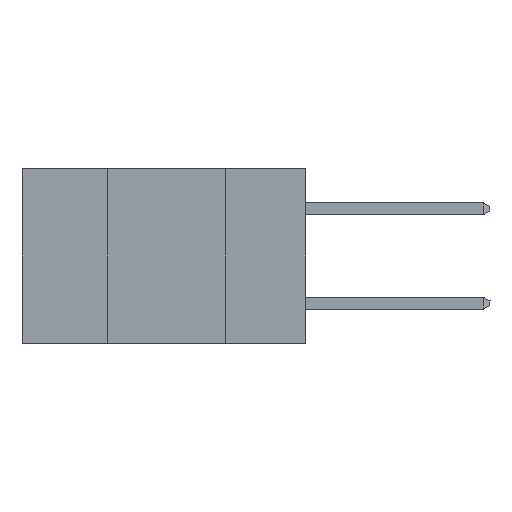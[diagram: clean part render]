
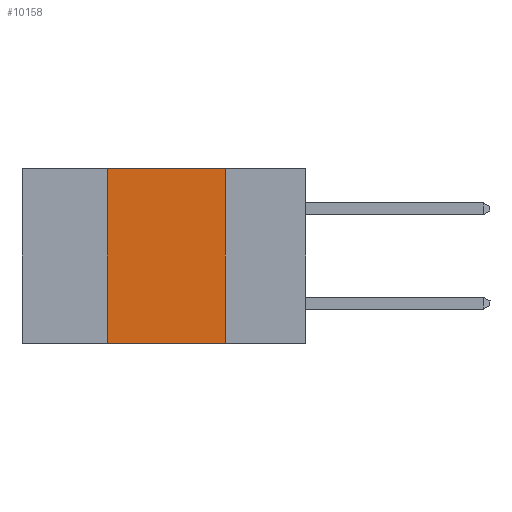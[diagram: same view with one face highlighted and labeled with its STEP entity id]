
A CAD part, left-side view. The second image highlights one B-rep face of the part: STEP entity #10158.
In plain terms, the highlighted planar face has unit normal (-1, 0, 0).
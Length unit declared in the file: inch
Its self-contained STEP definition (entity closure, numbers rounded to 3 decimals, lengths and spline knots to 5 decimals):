
#963 = DIRECTION ( 'NONE',  ( 0., 0., -1. ) ) ;
#1073 = VECTOR ( 'NONE', #13586, 39.37008 ) ;
#1571 = FACE_OUTER_BOUND ( 'NONE', #8847, .T. ) ;
#1975 = LINE ( 'NONE', #6987, #15641 ) ;
#2269 = DIRECTION ( 'NONE',  ( 1., 0., 0. ) ) ;
#4170 = CARTESIAN_POINT ( 'NONE',  ( 0., 0.42, -0.37 ) ) ;
#4775 = VECTOR ( 'NONE', #10990, 39.37008 ) ;
#5799 = ORIENTED_EDGE ( 'NONE', *, *, #15367, .F. ) ;
#5843 = CARTESIAN_POINT ( 'NONE',  ( 0., 0.6, 0. ) ) ;
#5894 = AXIS2_PLACEMENT_3D ( 'NONE', #5843, #2269, #5899 ) ;
#5899 = DIRECTION ( 'NONE',  ( 0., 0., -1. ) ) ;
#6035 = VERTEX_POINT ( 'NONE', #15513 ) ;
#6987 = CARTESIAN_POINT ( 'NONE',  ( 0., 0.42, 0. ) ) ;
#7324 = EDGE_CURVE ( 'NONE', #14330, #6035, #12401, .T. ) ;
#7697 = ORIENTED_EDGE ( 'NONE', *, *, #10081, .T. ) ;
#7794 = ORIENTED_EDGE ( 'NONE', *, *, #7915, .F. ) ;
#7915 = EDGE_CURVE ( 'NONE', #6035, #9547, #8115, .T. ) ;
#8115 = LINE ( 'NONE', #10890, #12366 ) ;
#8578 = PLANE ( 'NONE',  #5894 ) ;
#8752 = CARTESIAN_POINT ( 'NONE',  ( 0., 0.6, -0.37 ) ) ;
#8847 = EDGE_LOOP ( 'NONE', ( #7794, #11023, #5799, #7697 ) ) ;
#8922 = VERTEX_POINT ( 'NONE', #4170 ) ;
#9547 = VERTEX_POINT ( 'NONE', #10609 ) ;
#9777 = CARTESIAN_POINT ( 'NONE',  ( 0., 0.42, 0. ) ) ;
#10081 = EDGE_CURVE ( 'NONE', #8922, #9547, #13457, .T. ) ;
#10158 = ADVANCED_FACE ( 'NONE', ( #1571 ), #8578, .F. ) ;
#10609 = CARTESIAN_POINT ( 'NONE',  ( 0., 0.17, -0.37 ) ) ;
#10657 = DIRECTION ( 'NONE',  ( 0., 0., 1. ) ) ;
#10890 = CARTESIAN_POINT ( 'NONE',  ( 0., 0.17, 0. ) ) ;
#10990 = DIRECTION ( 'NONE',  ( 0., -1., 0. ) ) ;
#11018 = CARTESIAN_POINT ( 'NONE',  ( 0., 0.6, 0. ) ) ;
#11023 = ORIENTED_EDGE ( 'NONE', *, *, #7324, .F. ) ;
#12366 = VECTOR ( 'NONE', #963, 39.37008 ) ;
#12401 = LINE ( 'NONE', #11018, #1073 ) ;
#13457 = LINE ( 'NONE', #8752, #4775 ) ;
#13586 = DIRECTION ( 'NONE',  ( 0., -1., 0. ) ) ;
#14330 = VERTEX_POINT ( 'NONE', #9777 ) ;
#15367 = EDGE_CURVE ( 'NONE', #8922, #14330, #1975, .T. ) ;
#15513 = CARTESIAN_POINT ( 'NONE',  ( 0., 0.17, 0. ) ) ;
#15641 = VECTOR ( 'NONE', #10657, 39.37008 ) ;
